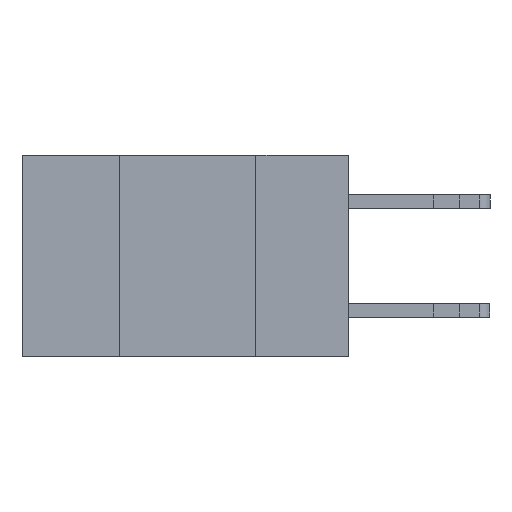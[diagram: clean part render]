
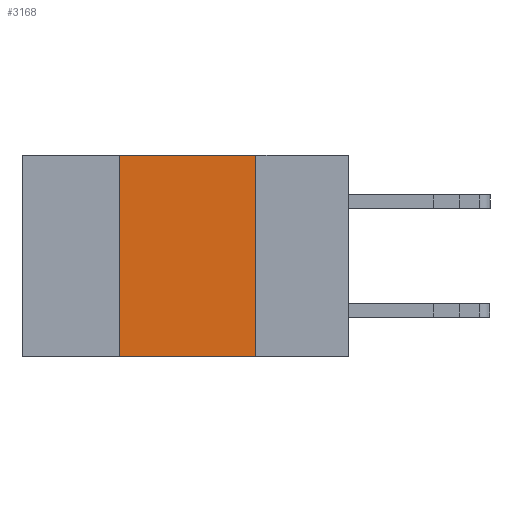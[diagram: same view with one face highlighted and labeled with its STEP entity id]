
A CAD part, left-side view. The second image highlights one B-rep face of the part: STEP entity #3168.
In plain terms, the highlighted planar face has unit normal (-1, 0, 0).
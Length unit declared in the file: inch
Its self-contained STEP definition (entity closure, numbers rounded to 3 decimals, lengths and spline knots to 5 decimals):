
#892 = CARTESIAN_POINT ( 'NONE',  ( 0., 0.42, -0.37 ) ) ;
#1197 = DIRECTION ( 'NONE',  ( 0., 0., -1. ) ) ;
#1502 = EDGE_LOOP ( 'NONE', ( #11894, #12101, #12442, #12822 ) ) ;
#2056 = CARTESIAN_POINT ( 'NONE',  ( 0., 0.17, 0. ) ) ;
#2241 = CARTESIAN_POINT ( 'NONE',  ( 0., 0.17, -0.37 ) ) ;
#2374 = VECTOR ( 'NONE', #14213, 39.37008 ) ;
#2382 = VERTEX_POINT ( 'NONE', #12172 ) ;
#2478 = DIRECTION ( 'NONE',  ( 0., -1., 0. ) ) ;
#2480 = LINE ( 'NONE', #10386, #11821 ) ;
#3168 = ADVANCED_FACE ( 'NONE', ( #10357 ), #3381, .F. ) ;
#3381 = PLANE ( 'NONE',  #8525 ) ;
#4009 = LINE ( 'NONE', #9376, #10042 ) ;
#4723 = EDGE_CURVE ( 'NONE', #5598, #6677, #2480, .T. ) ;
#5122 = CARTESIAN_POINT ( 'NONE',  ( 0., 0.6, 0. ) ) ;
#5598 = VERTEX_POINT ( 'NONE', #2056 ) ;
#5666 = LINE ( 'NONE', #5122, #14853 ) ;
#5848 = CARTESIAN_POINT ( 'NONE',  ( 0., 0.6, -0.37 ) ) ;
#5967 = VERTEX_POINT ( 'NONE', #892 ) ;
#6677 = VERTEX_POINT ( 'NONE', #2241 ) ;
#7097 = DIRECTION ( 'NONE',  ( 1., 0., 0. ) ) ;
#8525 = AXIS2_PLACEMENT_3D ( 'NONE', #9912, #7097, #1197 ) ;
#8786 = EDGE_CURVE ( 'NONE', #5967, #6677, #11727, .T. ) ;
#9376 = CARTESIAN_POINT ( 'NONE',  ( 0., 0.42, 0. ) ) ;
#9912 = CARTESIAN_POINT ( 'NONE',  ( 0., 0.6, 0. ) ) ;
#10042 = VECTOR ( 'NONE', #10568, 39.37008 ) ;
#10357 = FACE_OUTER_BOUND ( 'NONE', #1502, .T. ) ;
#10386 = CARTESIAN_POINT ( 'NONE',  ( 0., 0.17, 0. ) ) ;
#10568 = DIRECTION ( 'NONE',  ( 0., 0., 1. ) ) ;
#10620 = DIRECTION ( 'NONE',  ( 0., 0., -1. ) ) ;
#10919 = EDGE_CURVE ( 'NONE', #2382, #5598, #5666, .T. ) ;
#11727 = LINE ( 'NONE', #5848, #2374 ) ;
#11821 = VECTOR ( 'NONE', #10620, 39.37008 ) ;
#11894 = ORIENTED_EDGE ( 'NONE', *, *, #4723, .F. ) ;
#12101 = ORIENTED_EDGE ( 'NONE', *, *, #10919, .F. ) ;
#12172 = CARTESIAN_POINT ( 'NONE',  ( 0., 0.42, 0. ) ) ;
#12442 = ORIENTED_EDGE ( 'NONE', *, *, #13753, .F. ) ;
#12822 = ORIENTED_EDGE ( 'NONE', *, *, #8786, .T. ) ;
#13753 = EDGE_CURVE ( 'NONE', #5967, #2382, #4009, .T. ) ;
#14213 = DIRECTION ( 'NONE',  ( 0., -1., 0. ) ) ;
#14853 = VECTOR ( 'NONE', #2478, 39.37008 ) ;
